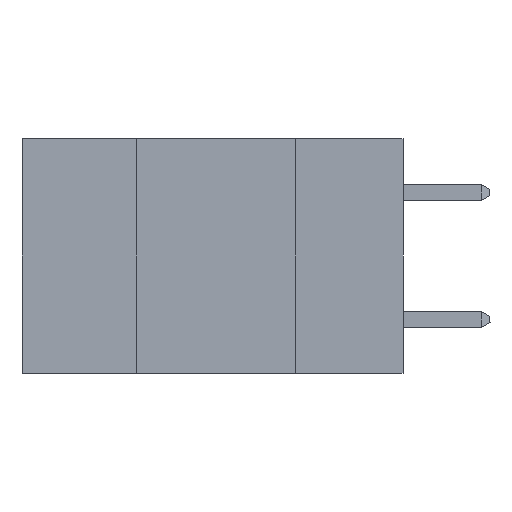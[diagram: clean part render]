
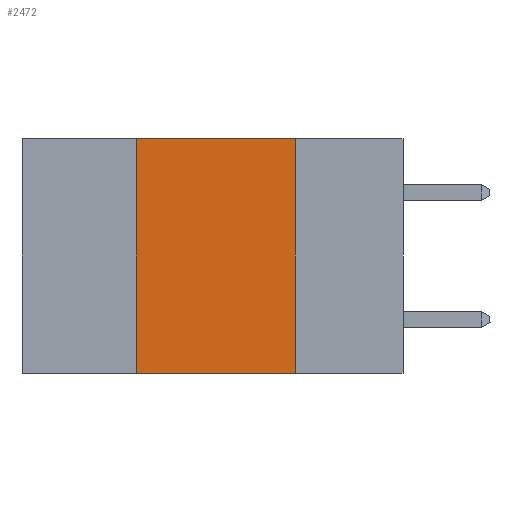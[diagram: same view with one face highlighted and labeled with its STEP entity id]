
A CAD part, left-side view. The second image highlights one B-rep face of the part: STEP entity #2472.
In plain terms, the highlighted planar face has unit normal (-1, 0, 0).
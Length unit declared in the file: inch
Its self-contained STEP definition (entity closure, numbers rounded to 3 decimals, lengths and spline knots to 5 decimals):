
#2472 = ADVANCED_FACE ( 'NONE', ( #4886 ), #16826, .F. ) ;
#4886 = FACE_OUTER_BOUND ( 'NONE', #21240, .T. ) ;
#8415 = CARTESIAN_POINT ( 'NONE',  ( 0., 0.17, 0. ) ) ;
#9545 = DIRECTION ( 'NONE',  ( 0., 0., -1. ) ) ;
#9856 = CARTESIAN_POINT ( 'NONE',  ( 0., 0.6, -0.37 ) ) ;
#11090 = VERTEX_POINT ( 'NONE', #8415 ) ;
#11305 = CARTESIAN_POINT ( 'NONE',  ( 0., 0.6, 0. ) ) ;
#11443 = VERTEX_POINT ( 'NONE', #12764 ) ;
#12590 = LINE ( 'NONE', #30257, #28698 ) ;
#12764 = CARTESIAN_POINT ( 'NONE',  ( 0., 0.42, -0.37 ) ) ;
#14849 = VECTOR ( 'NONE', #31403, 39.37008 ) ;
#15069 = ORIENTED_EDGE ( 'NONE', *, *, #18380, .F. ) ;
#16826 = PLANE ( 'NONE',  #19001 ) ;
#18380 = EDGE_CURVE ( 'NONE', #11443, #35469, #36193, .T. ) ;
#19001 = AXIS2_PLACEMENT_3D ( 'NONE', #34318, #31753, #31624 ) ;
#19071 = ORIENTED_EDGE ( 'NONE', *, *, #32904, .F. ) ;
#20977 = CARTESIAN_POINT ( 'NONE',  ( 0., 0.42, 0. ) ) ;
#21240 = EDGE_LOOP ( 'NONE', ( #37256, #19071, #15069, #27263 ) ) ;
#27263 = ORIENTED_EDGE ( 'NONE', *, *, #29869, .T. ) ;
#27461 = VERTEX_POINT ( 'NONE', #32338 ) ;
#27943 = VECTOR ( 'NONE', #35736, 39.37008 ) ;
#28215 = LINE ( 'NONE', #11305, #14849 ) ;
#28698 = VECTOR ( 'NONE', #9545, 39.37008 ) ;
#28779 = VECTOR ( 'NONE', #33656, 39.37008 ) ;
#29869 = EDGE_CURVE ( 'NONE', #11443, #27461, #37033, .T. ) ;
#30257 = CARTESIAN_POINT ( 'NONE',  ( 0., 0.17, 0. ) ) ;
#31403 = DIRECTION ( 'NONE',  ( 0., -1., 0. ) ) ;
#31624 = DIRECTION ( 'NONE',  ( 0., 0., -1. ) ) ;
#31753 = DIRECTION ( 'NONE',  ( 1., 0., 0. ) ) ;
#32338 = CARTESIAN_POINT ( 'NONE',  ( 0., 0.17, -0.37 ) ) ;
#32635 = EDGE_CURVE ( 'NONE', #11090, #27461, #12590, .T. ) ;
#32904 = EDGE_CURVE ( 'NONE', #35469, #11090, #28215, .T. ) ;
#33656 = DIRECTION ( 'NONE',  ( 0., -1., 0. ) ) ;
#34318 = CARTESIAN_POINT ( 'NONE',  ( 0., 0.6, 0. ) ) ;
#35469 = VERTEX_POINT ( 'NONE', #20977 ) ;
#35488 = CARTESIAN_POINT ( 'NONE',  ( 0., 0.42, 0. ) ) ;
#35736 = DIRECTION ( 'NONE',  ( 0., 0., 1. ) ) ;
#36193 = LINE ( 'NONE', #35488, #27943 ) ;
#37033 = LINE ( 'NONE', #9856, #28779 ) ;
#37256 = ORIENTED_EDGE ( 'NONE', *, *, #32635, .F. ) ;
